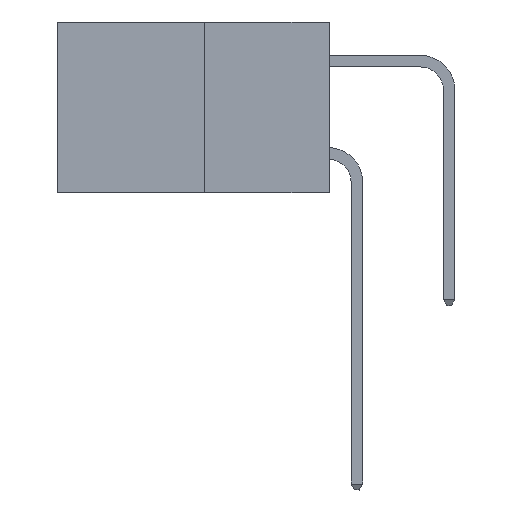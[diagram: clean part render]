
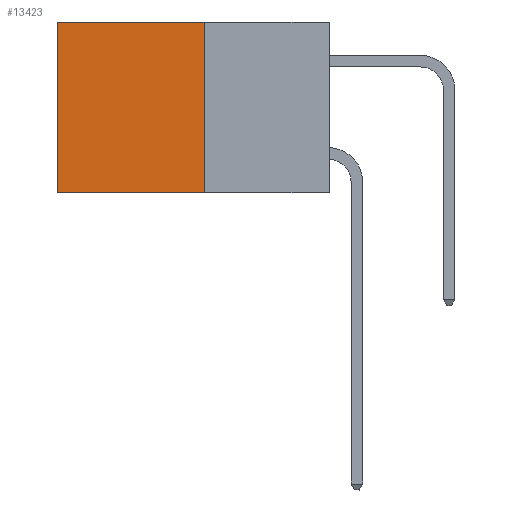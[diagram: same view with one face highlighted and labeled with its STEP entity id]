
A CAD part, left-side view. The second image highlights one B-rep face of the part: STEP entity #13423.
In plain terms, the highlighted planar face has unit normal (-1, 0, 0).
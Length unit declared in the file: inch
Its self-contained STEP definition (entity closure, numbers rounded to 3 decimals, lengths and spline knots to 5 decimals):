
#36 = DIRECTION ( 'NONE',  ( 1., 0., 0. ) ) ;
#499 = CARTESIAN_POINT ( 'NONE',  ( 0.277, 0.59, -0.37 ) ) ;
#649 = VERTEX_POINT ( 'NONE', #10210 ) ;
#686 = LINE ( 'NONE', #12680, #11949 ) ;
#1029 = LINE ( 'NONE', #2673, #8702 ) ;
#2673 = CARTESIAN_POINT ( 'NONE',  ( 0.277, 0.27, -0.37 ) ) ;
#2902 = VECTOR ( 'NONE', #13492, 39.37008 ) ;
#3577 = VERTEX_POINT ( 'NONE', #499 ) ;
#4970 = CARTESIAN_POINT ( 'NONE',  ( 0.277, 0.59, -0.37 ) ) ;
#5293 = EDGE_LOOP ( 'NONE', ( #16191, #12798, #6143, #6620 ) ) ;
#6143 = ORIENTED_EDGE ( 'NONE', *, *, #18224, .F. ) ;
#6205 = EDGE_CURVE ( 'NONE', #11224, #7449, #686, .T. ) ;
#6308 = FACE_OUTER_BOUND ( 'NONE', #5293, .T. ) ;
#6535 = DIRECTION ( 'NONE',  ( 0., 0., -1. ) ) ;
#6620 = ORIENTED_EDGE ( 'NONE', *, *, #6205, .T. ) ;
#7307 = AXIS2_PLACEMENT_3D ( 'NONE', #16654, #36, #10784 ) ;
#7328 = VECTOR ( 'NONE', #6535, 39.37008 ) ;
#7449 = VERTEX_POINT ( 'NONE', #13951 ) ;
#8702 = VECTOR ( 'NONE', #14874, 39.37008 ) ;
#8953 = CARTESIAN_POINT ( 'NONE',  ( 0.277, 0.27, -0.37 ) ) ;
#9248 = PLANE ( 'NONE',  #7307 ) ;
#10210 = CARTESIAN_POINT ( 'NONE',  ( 0.277, 0.27, -0.37 ) ) ;
#10784 = DIRECTION ( 'NONE',  ( 0., 0., -1. ) ) ;
#11224 = VERTEX_POINT ( 'NONE', #11849 ) ;
#11849 = CARTESIAN_POINT ( 'NONE',  ( 0.277, 0.27, 0. ) ) ;
#11949 = VECTOR ( 'NONE', #12639, 39.37008 ) ;
#12639 = DIRECTION ( 'NONE',  ( 0., 1., 0. ) ) ;
#12680 = CARTESIAN_POINT ( 'NONE',  ( 0.277, 0.27, 0. ) ) ;
#12798 = ORIENTED_EDGE ( 'NONE', *, *, #14034, .F. ) ;
#13423 = ADVANCED_FACE ( 'NONE', ( #6308 ), #9248, .F. ) ;
#13492 = DIRECTION ( 'NONE',  ( 0., 1., 0. ) ) ;
#13951 = CARTESIAN_POINT ( 'NONE',  ( 0.277, 0.59, 0. ) ) ;
#14034 = EDGE_CURVE ( 'NONE', #649, #3577, #14991, .T. ) ;
#14874 = DIRECTION ( 'NONE',  ( 0., 0., -1. ) ) ;
#14991 = LINE ( 'NONE', #8953, #2902 ) ;
#15319 = LINE ( 'NONE', #4970, #7328 ) ;
#16191 = ORIENTED_EDGE ( 'NONE', *, *, #17410, .T. ) ;
#16654 = CARTESIAN_POINT ( 'NONE',  ( 0.277, 0.27, -0.37 ) ) ;
#17410 = EDGE_CURVE ( 'NONE', #7449, #3577, #15319, .T. ) ;
#18224 = EDGE_CURVE ( 'NONE', #11224, #649, #1029, .T. ) ;
